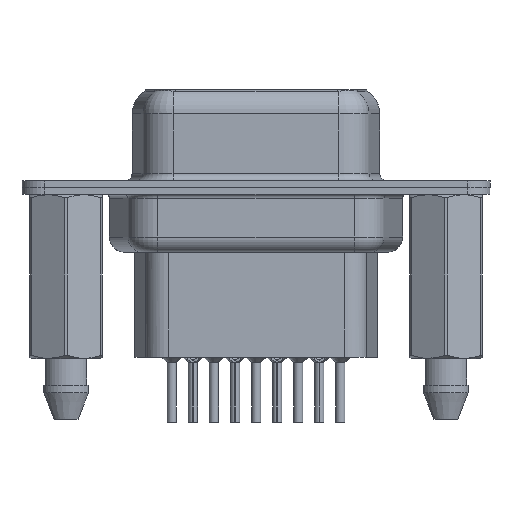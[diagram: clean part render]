
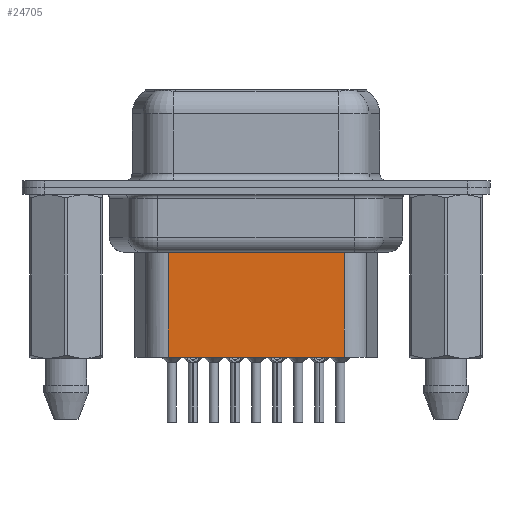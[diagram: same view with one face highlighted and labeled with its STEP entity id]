
A CAD part, front view. The second image highlights one B-rep face of the part: STEP entity #24705.
In plain terms, the highlighted planar face has unit normal (0, -1, 0).
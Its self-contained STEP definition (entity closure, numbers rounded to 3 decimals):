
#155 = DIRECTION ( 'NONE',  ( -1., 0., 0. ) ) ;
#252 = AXIS2_PLACEMENT_3D ( 'NONE', #13232, #9121, #14640 ) ;
#2462 = CARTESIAN_POINT ( 'NONE',  ( 6.459, -3.5, -4.097 ) ) ;
#2904 = ORIENTED_EDGE ( 'NONE', *, *, #4133, .F. ) ;
#3250 = PLANE ( 'NONE',  #252 ) ;
#3881 = DIRECTION ( 'NONE',  ( -1., 0., 0. ) ) ;
#4133 = EDGE_CURVE ( 'NONE', #24731, #8085, #13610, .T. ) ;
#5077 = LINE ( 'NONE', #18894, #20536 ) ;
#5694 = ORIENTED_EDGE ( 'NONE', *, *, #7986, .T. ) ;
#7888 = CARTESIAN_POINT ( 'NONE',  ( 18.294, -3.5, -4.097 ) ) ;
#7986 = EDGE_CURVE ( 'NONE', #20181, #8085, #9488, .T. ) ;
#8085 = VERTEX_POINT ( 'NONE', #14219 ) ;
#9121 = DIRECTION ( 'NONE',  ( 0., -1., 0. ) ) ;
#9488 = LINE ( 'NONE', #22943, #21151 ) ;
#9741 = EDGE_LOOP ( 'NONE', ( #20636, #13293, #5694, #2904 ) ) ;
#12180 = LINE ( 'NONE', #2462, #14646 ) ;
#12896 = DIRECTION ( 'NONE',  ( 0., 0., -1. ) ) ;
#12975 = FACE_OUTER_BOUND ( 'NONE', #9741, .T. ) ;
#13104 = CARTESIAN_POINT ( 'NONE',  ( 18.294, -3.5, -11.15 ) ) ;
#13232 = CARTESIAN_POINT ( 'NONE',  ( 6.706, -3.5, -3.1 ) ) ;
#13293 = ORIENTED_EDGE ( 'NONE', *, *, #20231, .T. ) ;
#13610 = LINE ( 'NONE', #19123, #16778 ) ;
#14219 = CARTESIAN_POINT ( 'NONE',  ( 6.706, -3.5, -11.15 ) ) ;
#14640 = DIRECTION ( 'NONE',  ( 1., 0., 0. ) ) ;
#14646 = VECTOR ( 'NONE', #155, 1000. ) ;
#15427 = VERTEX_POINT ( 'NONE', #7888 ) ;
#15975 = EDGE_CURVE ( 'NONE', #15427, #24731, #5077, .T. ) ;
#16778 = VECTOR ( 'NONE', #3881, 1000. ) ;
#18462 = CARTESIAN_POINT ( 'NONE',  ( 6.706, -3.5, -4.097 ) ) ;
#18894 = CARTESIAN_POINT ( 'NONE',  ( 18.294, -3.5, -3.1 ) ) ;
#19123 = CARTESIAN_POINT ( 'NONE',  ( 6.706, -3.5, -11.15 ) ) ;
#20181 = VERTEX_POINT ( 'NONE', #18462 ) ;
#20231 = EDGE_CURVE ( 'NONE', #15427, #20181, #12180, .T. ) ;
#20536 = VECTOR ( 'NONE', #12896, 1000. ) ;
#20636 = ORIENTED_EDGE ( 'NONE', *, *, #15975, .F. ) ;
#21151 = VECTOR ( 'NONE', #25131, 1000. ) ;
#22943 = CARTESIAN_POINT ( 'NONE',  ( 6.706, -3.5, -3.1 ) ) ;
#24705 = ADVANCED_FACE ( 'NONE', ( #12975 ), #3250, .T. ) ;
#24731 = VERTEX_POINT ( 'NONE', #13104 ) ;
#25131 = DIRECTION ( 'NONE',  ( 0., 0., -1. ) ) ;
